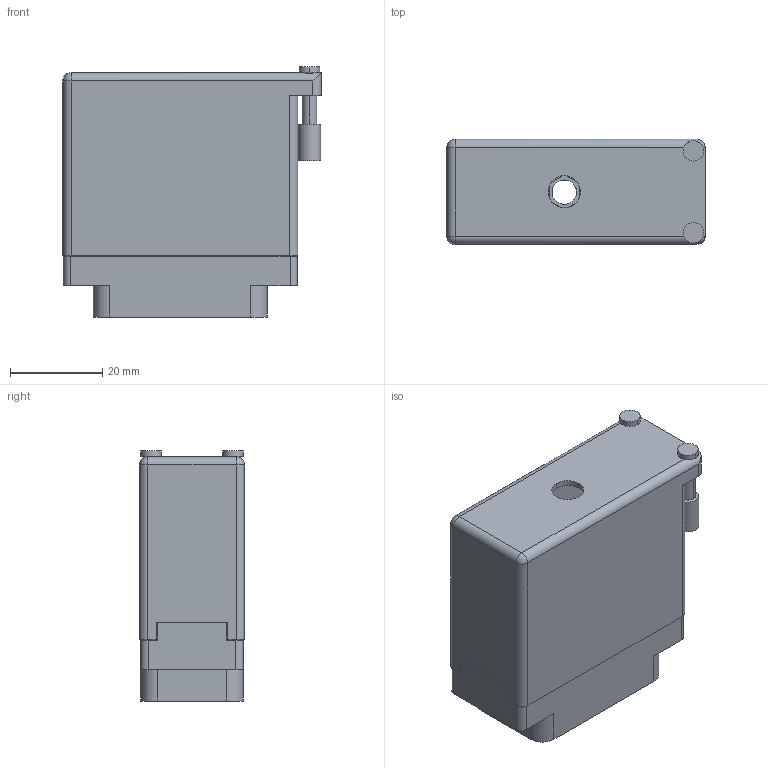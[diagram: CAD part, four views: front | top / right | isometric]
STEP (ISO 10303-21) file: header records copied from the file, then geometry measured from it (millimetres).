
FILE_DESCRIPTION (( 'STEP AP203' ), '1' );
FILE_NAME ('516-038-000-550.STEP', '2020-03-09T18:59:44', ( '' ), ( '' ), 'SwSTEP 2.0', 'SolidWorks 2016', '' );
FILE_SCHEMA (( 'CONFIG_CONTROL_DESIGN' ));
Length unit declared in the file: inch
Products named in the file (3): 516 Plug Insulator_038; 516-038-000-550; 516-230-001_Metal - 038 Side Entry
Assembly tree (2 placements, depth 2):
  516-038-000-550
    516 Plug Insulator_038
    516-230-001_Metal - 038 Side Entry
Bounding box: 56.08 x 22.83 x 54.31 mm (x, y, z)
Volume: 17426 mm3; surface area: 24980.1 mm2
Topology: 2 solids, 2 shells, 948 faces, 2767 edges, 1838 vertices
Faces by surface type: plane 674, cylinder 270, cone 2, sphere 2
Entity records: 31882 total; most frequent: CARTESIAN_POINT 5597, ORIENTED_EDGE 5530, DIRECTION 5355, EDGE_CURVE 2765, VECTOR 2071, LINE 2071, VERTEX_POINT 1838, AXIS2_PLACEMENT_3D 1642
